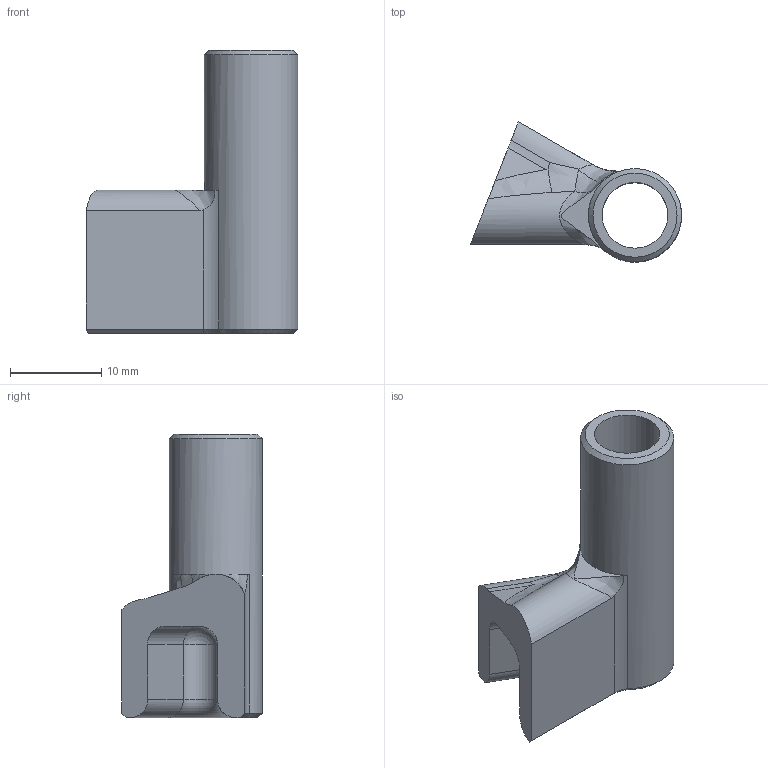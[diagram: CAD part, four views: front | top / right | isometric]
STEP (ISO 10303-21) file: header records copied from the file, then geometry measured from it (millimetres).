
FILE_DESCRIPTION(/* description */ (''),/* implementation_level */ '2;1');
FILE_NAME(/* name */ 'FGC-9_MkII_Recess_Jig.step',/* time_stamp */ '2021-03-24T22:32:43+01:00',/* author */ (''),/* organization */ (''),/* preprocessor_version */ 'ST-DEVELOPER v18.1',/* originating_system */ 'Autodesk Translation Framework v9.10.0.1330',/* authorisation */ '');
FILE_SCHEMA (('AUTOMOTIVE_DESIGN { 1 0 10303 214 3 1 1 }'));
Length unit declared in the file: millimetre
Products named in the file (2): FGC-9_MkII_Recess_Jig; FGC-9_MkII_Recess_Jig_1
Assembly tree (1 placements, depth 2):
  FGC-9_MkII_Recess_Jig
    FGC-9_MkII_Recess_Jig_1
Bounding box: 23.12 x 15.37 x 31 mm (x, y, z)
Volume: 2577.1 mm3; surface area: 2532.6 mm2
Topology: 1 solids, 1 shells, 37 faces, 94 edges, 59 vertices
Faces by surface type: cylinder 13, plane 12, bspline 7, cone 3, torus 1, sphere 1
Full cylindrical faces by diameter (mm): 7.2 x1, 10.2 x1
Entity records: 1483 total; most frequent: CARTESIAN_POINT 576, ORIENTED_EDGE 188, DIRECTION 168, EDGE_CURVE 94, AXIS2_PLACEMENT_3D 65, VERTEX_POINT 59, EDGE_LOOP 39, LINE 38
